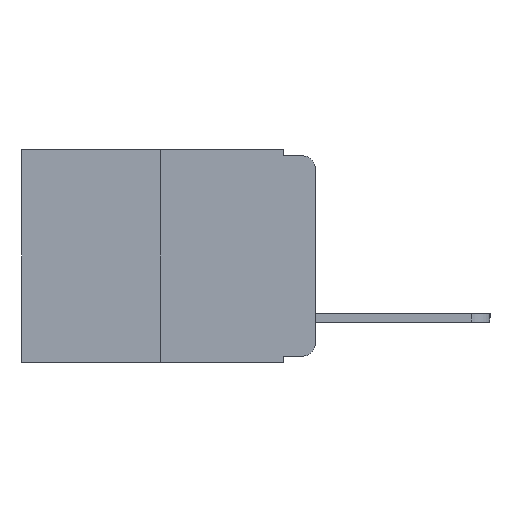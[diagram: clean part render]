
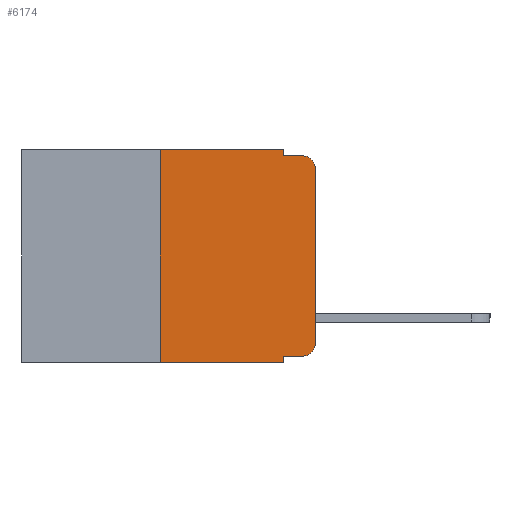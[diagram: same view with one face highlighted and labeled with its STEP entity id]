
A CAD part, left-side view. The second image highlights one B-rep face of the part: STEP entity #6174.
In plain terms, the highlighted planar face has unit normal (-1, 0, 0).
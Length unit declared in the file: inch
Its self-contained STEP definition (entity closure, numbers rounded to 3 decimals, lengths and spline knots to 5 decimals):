
#67 = ORIENTED_EDGE ( 'NONE', *, *, #5839, .T. ) ;
#168 = EDGE_CURVE ( 'NONE', #1676, #13160, #17167, .T. ) ;
#193 = DIRECTION ( 'NONE',  ( -1., 0., 0. ) ) ;
#558 = DIRECTION ( 'NONE',  ( 0., -1., 0. ) ) ;
#683 = VERTEX_POINT ( 'NONE', #15178 ) ;
#1338 = CARTESIAN_POINT ( 'NONE',  ( 0., 0.02, -0.313 ) ) ;
#1339 = ORIENTED_EDGE ( 'NONE', *, *, #8079, .F. ) ;
#1676 = VERTEX_POINT ( 'NONE', #5145 ) ;
#1714 = EDGE_CURVE ( 'NONE', #8127, #683, #13845, .T. ) ;
#2096 = CARTESIAN_POINT ( 'NONE',  ( 0., 0.051, -0.01 ) ) ;
#2219 = EDGE_CURVE ( 'NONE', #683, #17628, #9952, .T. ) ;
#2238 = VERTEX_POINT ( 'NONE', #3002 ) ;
#2336 = DIRECTION ( 'NONE',  ( 0., 0., -1. ) ) ;
#2339 = CARTESIAN_POINT ( 'NONE',  ( 0., 0.051, 0. ) ) ;
#2488 = CARTESIAN_POINT ( 'NONE',  ( 0., 0.051, 0. ) ) ;
#2513 = EDGE_CURVE ( 'NONE', #12802, #8958, #13237, .T. ) ;
#2519 = CARTESIAN_POINT ( 'NONE',  ( 0., 0.051, -0.333 ) ) ;
#2522 = ORIENTED_EDGE ( 'NONE', *, *, #168, .F. ) ;
#2736 = VECTOR ( 'NONE', #6733, 39.37008 ) ;
#2747 = ORIENTED_EDGE ( 'NONE', *, *, #4276, .T. ) ;
#3002 = CARTESIAN_POINT ( 'NONE',  ( 0., 0.051, -0.343 ) ) ;
#3694 = CARTESIAN_POINT ( 'NONE',  ( 0., 0.02, -0.01 ) ) ;
#4276 = EDGE_CURVE ( 'NONE', #17628, #9909, #10948, .T. ) ;
#4788 = LINE ( 'NONE', #15266, #11298 ) ;
#4994 = DIRECTION ( 'NONE',  ( 1., 0., 0. ) ) ;
#5051 = DIRECTION ( 'NONE',  ( 0., 0., -1. ) ) ;
#5055 = ORIENTED_EDGE ( 'NONE', *, *, #2513, .F. ) ;
#5145 = CARTESIAN_POINT ( 'NONE',  ( 0., 0.25, -0.343 ) ) ;
#5189 = CARTESIAN_POINT ( 'NONE',  ( 0., 0.051, -0.333 ) ) ;
#5244 = CIRCLE ( 'NONE', #15765, 0.02 ) ;
#5280 = DIRECTION ( 'NONE',  ( 0., 0., -1. ) ) ;
#5381 = CARTESIAN_POINT ( 'NONE',  ( 0., 0., 0. ) ) ;
#5839 = EDGE_CURVE ( 'NONE', #9909, #8958, #5244, .T. ) ;
#5895 = EDGE_CURVE ( 'NONE', #8127, #2238, #4788, .T. ) ;
#5990 = DIRECTION ( 'NONE',  ( 0., -1., 0. ) ) ;
#6174 = ADVANCED_FACE ( 'NONE', ( #17533 ), #14002, .F. ) ;
#6733 = DIRECTION ( 'NONE',  ( 0., 0., 1. ) ) ;
#6857 = CARTESIAN_POINT ( 'NONE',  ( 0., 0.473, 0. ) ) ;
#7136 = AXIS2_PLACEMENT_3D ( 'NONE', #6857, #4994, #5051 ) ;
#7285 = ORIENTED_EDGE ( 'NONE', *, *, #13287, .T. ) ;
#7643 = ORIENTED_EDGE ( 'NONE', *, *, #13150, .F. ) ;
#7930 = CARTESIAN_POINT ( 'NONE',  ( 0., 0.473, 0. ) ) ;
#8079 = EDGE_CURVE ( 'NONE', #13160, #11109, #14992, .T. ) ;
#8127 = VERTEX_POINT ( 'NONE', #5189 ) ;
#8191 = ORIENTED_EDGE ( 'NONE', *, *, #2219, .T. ) ;
#8378 = CARTESIAN_POINT ( 'NONE',  ( 0., 0.473, -0.343 ) ) ;
#8610 = VECTOR ( 'NONE', #17509, 39.37008 ) ;
#8768 = DIRECTION ( 'NONE',  ( 0., 0., 1. ) ) ;
#8958 = VERTEX_POINT ( 'NONE', #3694 ) ;
#9320 = VECTOR ( 'NONE', #11568, 39.37008 ) ;
#9857 = ORIENTED_EDGE ( 'NONE', *, *, #5895, .F. ) ;
#9909 = VERTEX_POINT ( 'NONE', #17698 ) ;
#9952 = CIRCLE ( 'NONE', #15204, 0.02 ) ;
#10364 = DIRECTION ( 'NONE',  ( 0., 0., -1. ) ) ;
#10391 = VECTOR ( 'NONE', #5990, 39.37008 ) ;
#10491 = ORIENTED_EDGE ( 'NONE', *, *, #1714, .T. ) ;
#10696 = VECTOR ( 'NONE', #5280, 39.37008 ) ;
#10948 = LINE ( 'NONE', #5381, #17413 ) ;
#11109 = VERTEX_POINT ( 'NONE', #2488 ) ;
#11157 = VECTOR ( 'NONE', #558, 39.37008 ) ;
#11298 = VECTOR ( 'NONE', #2336, 39.37008 ) ;
#11509 = DIRECTION ( 'NONE',  ( -1., 0., 0. ) ) ;
#11568 = DIRECTION ( 'NONE',  ( 0., -1., 0. ) ) ;
#12554 = LINE ( 'NONE', #8378, #8610 ) ;
#12802 = VERTEX_POINT ( 'NONE', #15340 ) ;
#13150 = EDGE_CURVE ( 'NONE', #11109, #12802, #14151, .T. ) ;
#13160 = VERTEX_POINT ( 'NONE', #17298 ) ;
#13237 = LINE ( 'NONE', #2096, #9320 ) ;
#13287 = EDGE_CURVE ( 'NONE', #1676, #2238, #12554, .T. ) ;
#13565 = CARTESIAN_POINT ( 'NONE',  ( 0., 0.25, 0. ) ) ;
#13845 = LINE ( 'NONE', #2519, #10391 ) ;
#14002 = PLANE ( 'NONE',  #7136 ) ;
#14151 = LINE ( 'NONE', #2339, #10696 ) ;
#14337 = CARTESIAN_POINT ( 'NONE',  ( 0., 0.02, -0.03 ) ) ;
#14350 = EDGE_LOOP ( 'NONE', ( #2747, #67, #5055, #7643, #1339, #2522, #7285, #9857, #10491, #8191 ) ) ;
#14992 = LINE ( 'NONE', #7930, #11157 ) ;
#15178 = CARTESIAN_POINT ( 'NONE',  ( 0., 0.02, -0.333 ) ) ;
#15204 = AXIS2_PLACEMENT_3D ( 'NONE', #1338, #11509, #17849 ) ;
#15266 = CARTESIAN_POINT ( 'NONE',  ( 0., 0.051, 0. ) ) ;
#15340 = CARTESIAN_POINT ( 'NONE',  ( 0., 0.051, -0.01 ) ) ;
#15765 = AXIS2_PLACEMENT_3D ( 'NONE', #14337, #193, #10364 ) ;
#16838 = CARTESIAN_POINT ( 'NONE',  ( 0., 0., -0.313 ) ) ;
#17167 = LINE ( 'NONE', #13565, #2736 ) ;
#17298 = CARTESIAN_POINT ( 'NONE',  ( 0., 0.25, 0. ) ) ;
#17413 = VECTOR ( 'NONE', #8768, 39.37008 ) ;
#17509 = DIRECTION ( 'NONE',  ( 0., -1., 0. ) ) ;
#17533 = FACE_OUTER_BOUND ( 'NONE', #14350, .T. ) ;
#17628 = VERTEX_POINT ( 'NONE', #16838 ) ;
#17698 = CARTESIAN_POINT ( 'NONE',  ( 0., 0., -0.03 ) ) ;
#17849 = DIRECTION ( 'NONE',  ( 0., 0., -1. ) ) ;
